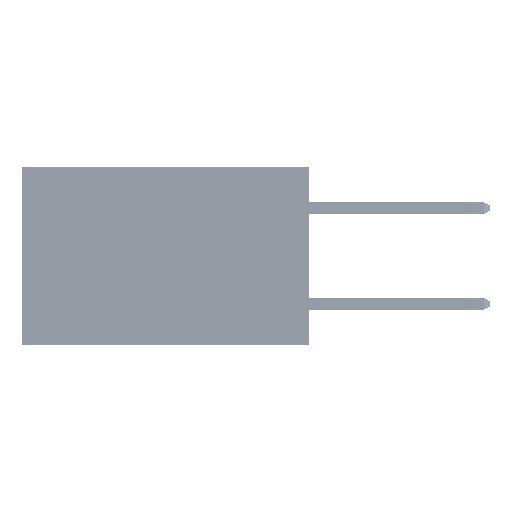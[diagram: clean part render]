
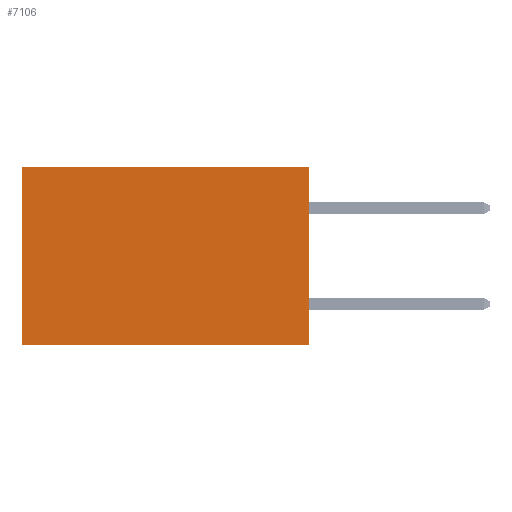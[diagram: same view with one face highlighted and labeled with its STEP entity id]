
A CAD part, left-side view. The second image highlights one B-rep face of the part: STEP entity #7106.
In plain terms, the highlighted planar face has unit normal (-1, 0, 0).
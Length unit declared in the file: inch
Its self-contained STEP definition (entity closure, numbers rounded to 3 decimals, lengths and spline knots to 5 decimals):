
#13 = VERTEX_POINT ( 'NONE', #36951 ) ;
#4205 = DIRECTION ( 'NONE',  ( 0., 1., 0. ) ) ;
#5815 = CARTESIAN_POINT ( 'NONE',  ( 0.2875, 0., 0. ) ) ;
#7106 = ADVANCED_FACE ( 'NONE', ( #7863 ), #7744, .F. ) ;
#7408 = DIRECTION ( 'NONE',  ( 0., 0., -1. ) ) ;
#7433 = EDGE_CURVE ( 'NONE', #14081, #36649, #16019, .T. ) ;
#7744 = PLANE ( 'NONE',  #11931 ) ;
#7863 = FACE_OUTER_BOUND ( 'NONE', #40953, .T. ) ;
#9100 = CARTESIAN_POINT ( 'NONE',  ( 0.2875, 0., -0.37 ) ) ;
#11931 = AXIS2_PLACEMENT_3D ( 'NONE', #37597, #26531, #7408 ) ;
#13457 = CARTESIAN_POINT ( 'NONE',  ( 0.2875, 0., 0. ) ) ;
#14081 = VERTEX_POINT ( 'NONE', #5815 ) ;
#15755 = VERTEX_POINT ( 'NONE', #42282 ) ;
#16019 = LINE ( 'NONE', #13457, #45771 ) ;
#16522 = CARTESIAN_POINT ( 'NONE',  ( 0.2875, 0.6, 0. ) ) ;
#19989 = LINE ( 'NONE', #37647, #27586 ) ;
#20294 = DIRECTION ( 'NONE',  ( 0., 0., -1. ) ) ;
#20857 = LINE ( 'NONE', #9100, #38319 ) ;
#21882 = ORIENTED_EDGE ( 'NONE', *, *, #32754, .T. ) ;
#24218 = EDGE_CURVE ( 'NONE', #36649, #15755, #20857, .T. ) ;
#26531 = DIRECTION ( 'NONE',  ( 1., 0., 0. ) ) ;
#27586 = VECTOR ( 'NONE', #4205, 39.37008 ) ;
#31156 = DIRECTION ( 'NONE',  ( 0., 1., 0. ) ) ;
#31962 = EDGE_CURVE ( 'NONE', #13, #15755, #45509, .T. ) ;
#32754 = EDGE_CURVE ( 'NONE', #14081, #13, #19989, .T. ) ;
#33128 = CARTESIAN_POINT ( 'NONE',  ( 0.2875, 0., -0.37 ) ) ;
#35592 = ORIENTED_EDGE ( 'NONE', *, *, #7433, .F. ) ;
#35941 = ORIENTED_EDGE ( 'NONE', *, *, #24218, .F. ) ;
#36649 = VERTEX_POINT ( 'NONE', #33128 ) ;
#36951 = CARTESIAN_POINT ( 'NONE',  ( 0.2875, 0.6, 0. ) ) ;
#37597 = CARTESIAN_POINT ( 'NONE',  ( 0.2875, 0., 0. ) ) ;
#37647 = CARTESIAN_POINT ( 'NONE',  ( 0.2875, 0., 0. ) ) ;
#38319 = VECTOR ( 'NONE', #31156, 39.37008 ) ;
#40840 = DIRECTION ( 'NONE',  ( 0., 0., -1. ) ) ;
#40953 = EDGE_LOOP ( 'NONE', ( #45304, #35941, #35592, #21882 ) ) ;
#42282 = CARTESIAN_POINT ( 'NONE',  ( 0.2875, 0.6, -0.37 ) ) ;
#42819 = VECTOR ( 'NONE', #20294, 39.37008 ) ;
#45304 = ORIENTED_EDGE ( 'NONE', *, *, #31962, .T. ) ;
#45509 = LINE ( 'NONE', #16522, #42819 ) ;
#45771 = VECTOR ( 'NONE', #40840, 39.37008 ) ;
